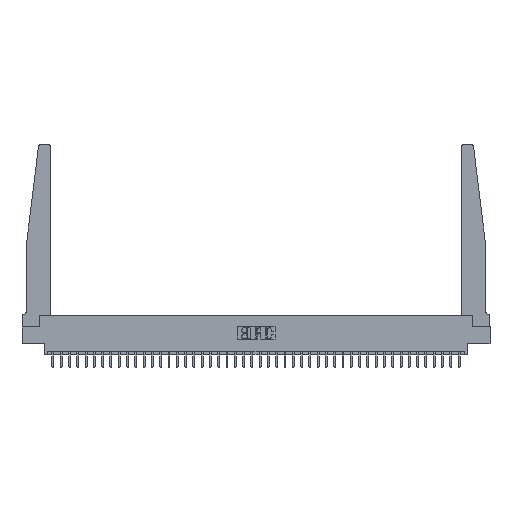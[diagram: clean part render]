
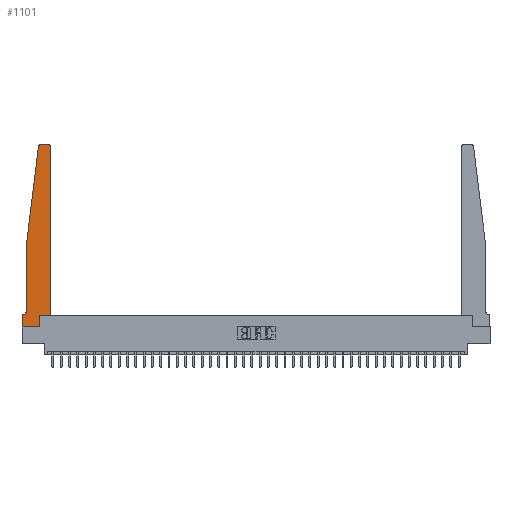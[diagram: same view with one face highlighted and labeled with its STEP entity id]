
A CAD part, top view. The second image highlights one B-rep face of the part: STEP entity #1101.
In plain terms, the highlighted planar face has unit normal (0, 0, 1).
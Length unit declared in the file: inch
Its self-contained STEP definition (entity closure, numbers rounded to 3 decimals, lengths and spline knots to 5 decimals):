
#236 = VERTEX_POINT ( 'NONE', #27529 ) ;
#645 = VERTEX_POINT ( 'NONE', #18060 ) ;
#1101 = ADVANCED_FACE ( 'NONE', ( #34642 ), #8365, .T. ) ;
#1299 = DIRECTION ( 'NONE',  ( 0., 1., 0. ) ) ;
#1775 = EDGE_CURVE ( 'NONE', #5401, #19755, #24240, .T. ) ;
#1908 = LINE ( 'NONE', #9090, #14590 ) ;
#2047 = VERTEX_POINT ( 'NONE', #4925 ) ;
#2449 = AXIS2_PLACEMENT_3D ( 'NONE', #31876, #15128, #34620 ) ;
#3780 = AXIS2_PLACEMENT_3D ( 'NONE', #28190, #31011, #14245 ) ;
#3790 = DIRECTION ( 'NONE',  ( 0., -1., 0. ) ) ;
#4033 = EDGE_CURVE ( 'NONE', #36508, #33603, #35762, .T. ) ;
#4084 = CARTESIAN_POINT ( 'NONE',  ( 0.425, 0.18, 0.37 ) ) ;
#4188 = VECTOR ( 'NONE', #28600, 39.37008 ) ;
#4660 = CIRCLE ( 'NONE', #2449, 0.03 ) ;
#4925 = CARTESIAN_POINT ( 'NONE',  ( 0., 0.1875, 0.37 ) ) ;
#5181 = DIRECTION ( 'NONE',  ( -1., 0., 0. ) ) ;
#5321 = ORIENTED_EDGE ( 'NONE', *, *, #4033, .T. ) ;
#5401 = VERTEX_POINT ( 'NONE', #30433 ) ;
#5907 = CARTESIAN_POINT ( 'NONE',  ( 0.425, 0.18, 0.37 ) ) ;
#6549 = ORIENTED_EDGE ( 'NONE', *, *, #7550, .T. ) ;
#6589 = CARTESIAN_POINT ( 'NONE',  ( 0., 0., 0.37 ) ) ;
#6958 = CARTESIAN_POINT ( 'NONE',  ( 0.425, 2.72, 0.37 ) ) ;
#7208 = LINE ( 'NONE', #18100, #21524 ) ;
#7550 = EDGE_CURVE ( 'NONE', #33603, #10269, #4660, .T. ) ;
#7562 = AXIS2_PLACEMENT_3D ( 'NONE', #13697, #33281, #16569 ) ;
#8124 = AXIS2_PLACEMENT_3D ( 'NONE', #11248, #30970, #14202 ) ;
#8365 = PLANE ( 'NONE',  #3780 ) ;
#8483 = VECTOR ( 'NONE', #1299, 39.37008 ) ;
#9090 = CARTESIAN_POINT ( 'NONE',  ( 0.065, 0.1875, 0.37 ) ) ;
#9388 = CARTESIAN_POINT ( 'NONE',  ( 0.015, 0.1875, 0.37 ) ) ;
#9460 = VERTEX_POINT ( 'NONE', #17503 ) ;
#9683 = ORIENTED_EDGE ( 'NONE', *, *, #12503, .T. ) ;
#10269 = VERTEX_POINT ( 'NONE', #18684 ) ;
#10522 = VECTOR ( 'NONE', #23326, 39.37008 ) ;
#10554 = ORIENTED_EDGE ( 'NONE', *, *, #31151, .T. ) ;
#11248 = CARTESIAN_POINT ( 'NONE',  ( 0.015, 0.2375, 0.37 ) ) ;
#11439 = LINE ( 'NONE', #31641, #10522 ) ;
#11507 = EDGE_CURVE ( 'NONE', #2047, #12022, #27232, .T. ) ;
#11554 = CIRCLE ( 'NONE', #7562, 0.03 ) ;
#12022 = VERTEX_POINT ( 'NONE', #23446 ) ;
#12103 = DIRECTION ( 'NONE',  ( 0., -1., 0. ) ) ;
#12503 = EDGE_CURVE ( 'NONE', #10269, #645, #13586, .T. ) ;
#12576 = VECTOR ( 'NONE', #5181, 39.37008 ) ;
#12657 = VECTOR ( 'NONE', #19752, 39.37008 ) ;
#12787 = EDGE_CURVE ( 'NONE', #12022, #236, #33701, .T. ) ;
#12871 = VERTEX_POINT ( 'NONE', #6958 ) ;
#13205 = ORIENTED_EDGE ( 'NONE', *, *, #1775, .T. ) ;
#13351 = ORIENTED_EDGE ( 'NONE', *, *, #18329, .T. ) ;
#13586 = LINE ( 'NONE', #25275, #12657 ) ;
#13697 = CARTESIAN_POINT ( 'NONE',  ( 0.395, 2.72, 0.37 ) ) ;
#14202 = DIRECTION ( 'NONE',  ( -1., 0., 0. ) ) ;
#14245 = DIRECTION ( 'NONE',  ( 1., 0., 0. ) ) ;
#14590 = VECTOR ( 'NONE', #34347, 39.37008 ) ;
#15128 = DIRECTION ( 'NONE',  ( 0., 0., 1. ) ) ;
#15357 = EDGE_LOOP ( 'NONE', ( #5321, #6549, #9683, #10554, #13205, #13351, #21756, #22918, #29191, #29262, #34123, #34303 ) ) ;
#16208 = LINE ( 'NONE', #4084, #8483 ) ;
#16551 = CARTESIAN_POINT ( 'NONE',  ( 0.25, 2.75, 0.37 ) ) ;
#16569 = DIRECTION ( 'NONE',  ( 1., 0., 0. ) ) ;
#17503 = CARTESIAN_POINT ( 'NONE',  ( 0.2605, 0.18, 0.37 ) ) ;
#18060 = CARTESIAN_POINT ( 'NONE',  ( 0.065, 1.25, 0.37 ) ) ;
#18100 = CARTESIAN_POINT ( 'NONE',  ( 0.065, 1.25, 0.37 ) ) ;
#18329 = EDGE_CURVE ( 'NONE', #19755, #2047, #1908, .T. ) ;
#18684 = CARTESIAN_POINT ( 'NONE',  ( 0.24675, 2.72367, 0.37 ) ) ;
#19590 = VERTEX_POINT ( 'NONE', #31263 ) ;
#19752 = DIRECTION ( 'NONE',  ( -0.122, -0.992, 0. ) ) ;
#19755 = VERTEX_POINT ( 'NONE', #9388 ) ;
#21524 = VECTOR ( 'NONE', #3790, 39.37008 ) ;
#21756 = ORIENTED_EDGE ( 'NONE', *, *, #11507, .T. ) ;
#22842 = EDGE_CURVE ( 'NONE', #12871, #36508, #11554, .T. ) ;
#22918 = ORIENTED_EDGE ( 'NONE', *, *, #12787, .T. ) ;
#23326 = DIRECTION ( 'NONE',  ( 0., 1., 0. ) ) ;
#23446 = CARTESIAN_POINT ( 'NONE',  ( 0., 0., 0.37 ) ) ;
#23766 = DIRECTION ( 'NONE',  ( 1., 0., 0. ) ) ;
#24240 = CIRCLE ( 'NONE', #8124, 0.05 ) ;
#25275 = CARTESIAN_POINT ( 'NONE',  ( 0.065, 1.25, 0.37 ) ) ;
#26202 = CARTESIAN_POINT ( 'NONE',  ( 0., 0., 0.37 ) ) ;
#26335 = VECTOR ( 'NONE', #23766, 39.37008 ) ;
#27232 = LINE ( 'NONE', #26202, #33724 ) ;
#27529 = CARTESIAN_POINT ( 'NONE',  ( 0.2605, 0., 0.37 ) ) ;
#28190 = CARTESIAN_POINT ( 'NONE',  ( 0., 0.1875, 0.37 ) ) ;
#28600 = DIRECTION ( 'NONE',  ( 1., 0., 0. ) ) ;
#29191 = ORIENTED_EDGE ( 'NONE', *, *, #31789, .T. ) ;
#29262 = ORIENTED_EDGE ( 'NONE', *, *, #32004, .T. ) ;
#30433 = CARTESIAN_POINT ( 'NONE',  ( 0.065, 0.2375, 0.37 ) ) ;
#30970 = DIRECTION ( 'NONE',  ( 0., 0., -1. ) ) ;
#31011 = DIRECTION ( 'NONE',  ( 0., 0., 1. ) ) ;
#31151 = EDGE_CURVE ( 'NONE', #645, #5401, #7208, .T. ) ;
#31263 = CARTESIAN_POINT ( 'NONE',  ( 0.425, 0.18, 0.37 ) ) ;
#31641 = CARTESIAN_POINT ( 'NONE',  ( 0.2605, 0.18, 0.37 ) ) ;
#31789 = EDGE_CURVE ( 'NONE', #236, #9460, #11439, .T. ) ;
#31876 = CARTESIAN_POINT ( 'NONE',  ( 0.27653, 2.72, 0.37 ) ) ;
#32004 = EDGE_CURVE ( 'NONE', #9460, #19590, #34273, .T. ) ;
#33281 = DIRECTION ( 'NONE',  ( 0., 0., 1. ) ) ;
#33603 = VERTEX_POINT ( 'NONE', #35259 ) ;
#33701 = LINE ( 'NONE', #6589, #26335 ) ;
#33724 = VECTOR ( 'NONE', #12103, 39.37008 ) ;
#34123 = ORIENTED_EDGE ( 'NONE', *, *, #34655, .T. ) ;
#34273 = LINE ( 'NONE', #5907, #4188 ) ;
#34303 = ORIENTED_EDGE ( 'NONE', *, *, #22842, .T. ) ;
#34347 = DIRECTION ( 'NONE',  ( -1., 0., 0. ) ) ;
#34463 = CARTESIAN_POINT ( 'NONE',  ( 0.395, 2.75, 0.37 ) ) ;
#34620 = DIRECTION ( 'NONE',  ( 1., 0., 0. ) ) ;
#34642 = FACE_OUTER_BOUND ( 'NONE', #15357, .T. ) ;
#34655 = EDGE_CURVE ( 'NONE', #19590, #12871, #16208, .T. ) ;
#35259 = CARTESIAN_POINT ( 'NONE',  ( 0.27653, 2.75, 0.37 ) ) ;
#35762 = LINE ( 'NONE', #16551, #12576 ) ;
#36508 = VERTEX_POINT ( 'NONE', #34463 ) ;
